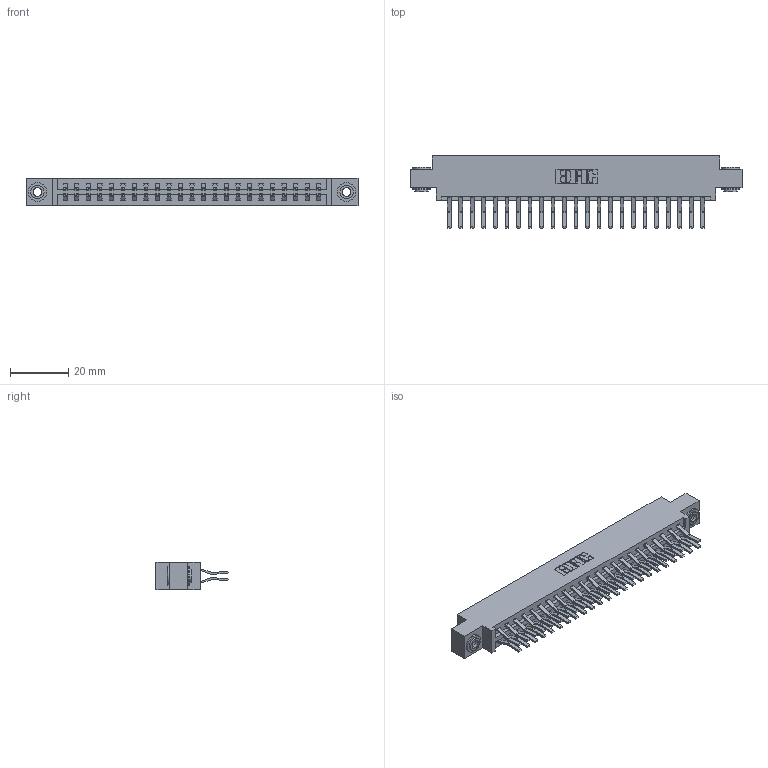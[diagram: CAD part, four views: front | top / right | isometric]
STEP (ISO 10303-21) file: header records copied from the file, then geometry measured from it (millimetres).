
FILE_DESCRIPTION (( 'STEP AP203' ), '1' );
FILE_NAME ('337-046-560-803.STEP', '2019-10-11T15:00:44', ( '' ), ( '' ), 'SwSTEP 2.0', 'SolidWorks 2016', '' );
FILE_SCHEMA (( 'CONFIG_CONTROL_DESIGN' ));
Length unit declared in the file: inch
Products named in the file (4): 345-250-002_345-250-002-102; 337-046-560-803; 337 Part_0.170 Offset - 0.156 Dia-TH; 345-292-001_560 Tail
Assembly tree (49 placements, depth 2):
  337-046-560-803
    337 Part_0.170 Offset - 0.156 Dia-TH
    345-292-001_560 Tail  x46
    345-250-002_345-250-002-102  x2
Bounding box: 114.15 x 24.78 x 9.4 mm (x, y, z)
Volume: 11980.3 mm3; surface area: 14564 mm2
Topology: 49 solids, 49 shells, 2732 faces, 8081 edges, 5322 vertices
Faces by surface type: plane 1832, cylinder 892, cone 8
Entity records: 21160 total; most frequent: CARTESIAN_POINT 3557, ORIENTED_EDGE 3486, DIRECTION 3097, EDGE_CURVE 1743, LINE 1587, VECTOR 1587, VERTEX_POINT 1158, AXIS2_PLACEMENT_3D 755
